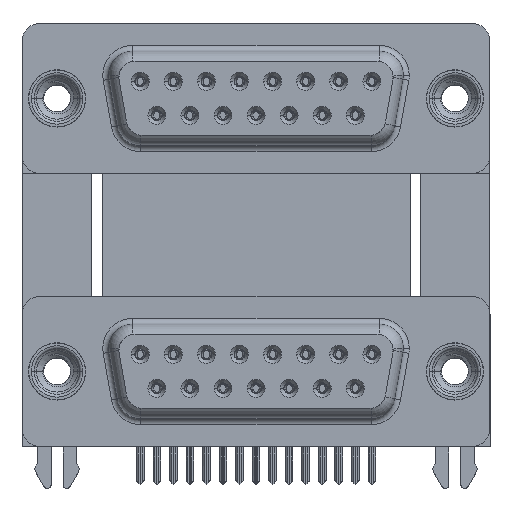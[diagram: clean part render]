
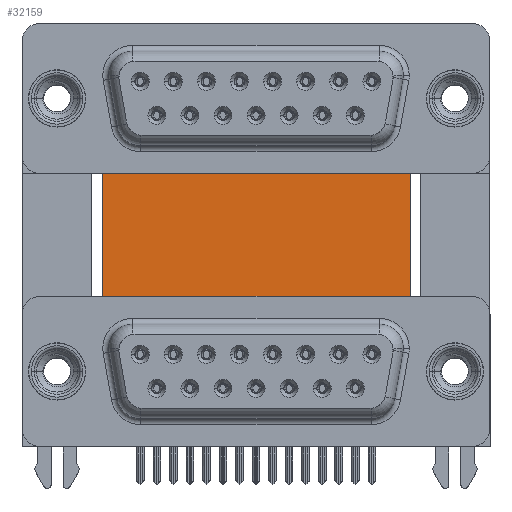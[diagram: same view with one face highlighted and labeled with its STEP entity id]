
A CAD part, top view. The second image highlights one B-rep face of the part: STEP entity #32159.
In plain terms, the highlighted planar face has unit normal (0, 0, 1).
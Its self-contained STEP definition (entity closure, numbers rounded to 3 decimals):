
#1173 = CARTESIAN_POINT ( 'NONE',  ( 3.79, -3.735, -12. ) ) ;
#3152 = VERTEX_POINT ( 'NONE', #38400 ) ;
#3349 = DIRECTION ( 'NONE',  ( 1., 0., 0. ) ) ;
#4418 = AXIS2_PLACEMENT_3D ( 'NONE', #46010, #26247, #42080 ) ;
#5147 = VERTEX_POINT ( 'NONE', #20905 ) ;
#6202 = FACE_OUTER_BOUND ( 'NONE', #35482, .T. ) ;
#6607 = LINE ( 'NONE', #30549, #31682 ) ;
#7551 = ORIENTED_EDGE ( 'NONE', *, *, #9422, .T. ) ;
#9422 = EDGE_CURVE ( 'NONE', #35473, #5147, #13154, .T. ) ;
#10604 = CARTESIAN_POINT ( 'NONE',  ( 29.58, 16.585, -12. ) ) ;
#10793 = VECTOR ( 'NONE', #38591, 1000. ) ;
#11146 = CARTESIAN_POINT ( 'NONE',  ( 3.79, 16.585, -12. ) ) ;
#13154 = LINE ( 'NONE', #1173, #23038 ) ;
#13416 = DIRECTION ( 'NONE',  ( 1., 0., 0. ) ) ;
#15524 = CARTESIAN_POINT ( 'NONE',  ( 3.79, -3.735, -12. ) ) ;
#15966 = ORIENTED_EDGE ( 'NONE', *, *, #28484, .F. ) ;
#18312 = LINE ( 'NONE', #38081, #10793 ) ;
#20266 = ORIENTED_EDGE ( 'NONE', *, *, #24322, .F. ) ;
#20905 = CARTESIAN_POINT ( 'NONE',  ( 29.58, -3.735, -12. ) ) ;
#22083 = PLANE ( 'NONE',  #4418 ) ;
#23038 = VECTOR ( 'NONE', #13416, 1000. ) ;
#24322 = EDGE_CURVE ( 'NONE', #3152, #27724, #26289, .T. ) ;
#26247 = DIRECTION ( 'NONE',  ( 0., 0., -1. ) ) ;
#26289 = LINE ( 'NONE', #11146, #51389 ) ;
#27724 = VERTEX_POINT ( 'NONE', #10604 ) ;
#28484 = EDGE_CURVE ( 'NONE', #27724, #5147, #18312, .T. ) ;
#29608 = EDGE_CURVE ( 'NONE', #3152, #35473, #6607, .T. ) ;
#30549 = CARTESIAN_POINT ( 'NONE',  ( 3.79, 16.585, -12. ) ) ;
#31682 = VECTOR ( 'NONE', #41471, 1000. ) ;
#32159 = ADVANCED_FACE ( 'NONE', ( #6202 ), #22083, .F. ) ;
#34994 = ORIENTED_EDGE ( 'NONE', *, *, #29608, .T. ) ;
#35473 = VERTEX_POINT ( 'NONE', #15524 ) ;
#35482 = EDGE_LOOP ( 'NONE', ( #7551, #15966, #20266, #34994 ) ) ;
#38081 = CARTESIAN_POINT ( 'NONE',  ( 29.58, 16.585, -12. ) ) ;
#38400 = CARTESIAN_POINT ( 'NONE',  ( 3.79, 16.585, -12. ) ) ;
#38591 = DIRECTION ( 'NONE',  ( 0., -1., 0. ) ) ;
#41471 = DIRECTION ( 'NONE',  ( 0., -1., 0. ) ) ;
#42080 = DIRECTION ( 'NONE',  ( -1., 0., 0. ) ) ;
#46010 = CARTESIAN_POINT ( 'NONE',  ( 3.79, 16.585, -12. ) ) ;
#51389 = VECTOR ( 'NONE', #3349, 1000. ) ;
